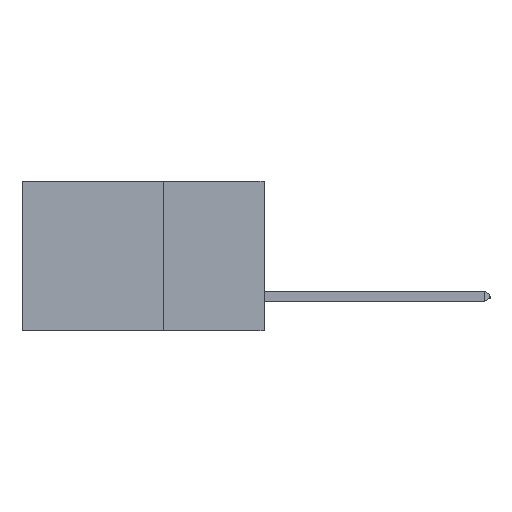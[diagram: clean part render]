
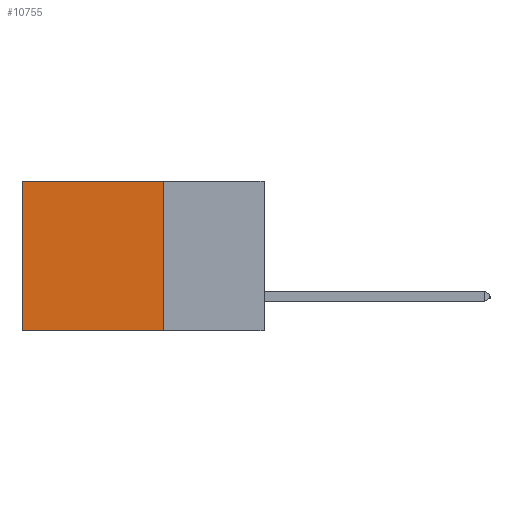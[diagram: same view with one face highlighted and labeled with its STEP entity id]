
A CAD part, left-side view. The second image highlights one B-rep face of the part: STEP entity #10755.
In plain terms, the highlighted planar face has unit normal (-1, 0, 0).
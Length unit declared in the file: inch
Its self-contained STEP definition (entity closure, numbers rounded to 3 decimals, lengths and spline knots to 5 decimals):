
#171 = CARTESIAN_POINT ( 'NONE',  ( 0.298, 0.25, 0. ) ) ;
#355 = CARTESIAN_POINT ( 'NONE',  ( 0.298, 0.25, 0. ) ) ;
#556 = CARTESIAN_POINT ( 'NONE',  ( 0.298, 0.25, 0. ) ) ;
#808 = LINE ( 'NONE', #355, #17858 ) ;
#933 = LINE ( 'NONE', #8354, #17980 ) ;
#1272 = LINE ( 'NONE', #556, #13489 ) ;
#1714 = FACE_OUTER_BOUND ( 'NONE', #8327, .T. ) ;
#2478 = ORIENTED_EDGE ( 'NONE', *, *, #3419, .T. ) ;
#3123 = VERTEX_POINT ( 'NONE', #16692 ) ;
#3419 = EDGE_CURVE ( 'NONE', #6605, #6848, #1272, .T. ) ;
#3555 = VECTOR ( 'NONE', #7746, 39.37008 ) ;
#4523 = DIRECTION ( 'NONE',  ( 0., 1., 0. ) ) ;
#5250 = PLANE ( 'NONE',  #12853 ) ;
#6605 = VERTEX_POINT ( 'NONE', #171 ) ;
#6848 = VERTEX_POINT ( 'NONE', #9298 ) ;
#7180 = DIRECTION ( 'NONE',  ( 0., 0., -1. ) ) ;
#7746 = DIRECTION ( 'NONE',  ( 0., 0., -1. ) ) ;
#8327 = EDGE_LOOP ( 'NONE', ( #20099, #15583, #15756, #2478 ) ) ;
#8354 = CARTESIAN_POINT ( 'NONE',  ( 0.298, 0.25, -0.37 ) ) ;
#8587 = DIRECTION ( 'NONE',  ( 1., 0., 0. ) ) ;
#9298 = CARTESIAN_POINT ( 'NONE',  ( 0.298, 0.6, 0. ) ) ;
#10755 = ADVANCED_FACE ( 'NONE', ( #1714 ), #5250, .F. ) ;
#11077 = CARTESIAN_POINT ( 'NONE',  ( 0.298, 0.6, -0.37 ) ) ;
#12853 = AXIS2_PLACEMENT_3D ( 'NONE', #15036, #8587, #19885 ) ;
#13489 = VECTOR ( 'NONE', #4523, 39.37008 ) ;
#14418 = EDGE_CURVE ( 'NONE', #3123, #17559, #933, .T. ) ;
#15036 = CARTESIAN_POINT ( 'NONE',  ( 0.298, 0.25, 0. ) ) ;
#15583 = ORIENTED_EDGE ( 'NONE', *, *, #14418, .F. ) ;
#15756 = ORIENTED_EDGE ( 'NONE', *, *, #19676, .F. ) ;
#16398 = DIRECTION ( 'NONE',  ( 0., 1., 0. ) ) ;
#16628 = LINE ( 'NONE', #20598, #3555 ) ;
#16692 = CARTESIAN_POINT ( 'NONE',  ( 0.298, 0.25, -0.37 ) ) ;
#17519 = EDGE_CURVE ( 'NONE', #6848, #17559, #16628, .T. ) ;
#17559 = VERTEX_POINT ( 'NONE', #11077 ) ;
#17858 = VECTOR ( 'NONE', #7180, 39.37008 ) ;
#17980 = VECTOR ( 'NONE', #16398, 39.37008 ) ;
#19676 = EDGE_CURVE ( 'NONE', #6605, #3123, #808, .T. ) ;
#19885 = DIRECTION ( 'NONE',  ( 0., 0., -1. ) ) ;
#20099 = ORIENTED_EDGE ( 'NONE', *, *, #17519, .T. ) ;
#20598 = CARTESIAN_POINT ( 'NONE',  ( 0.298, 0.6, 0. ) ) ;
